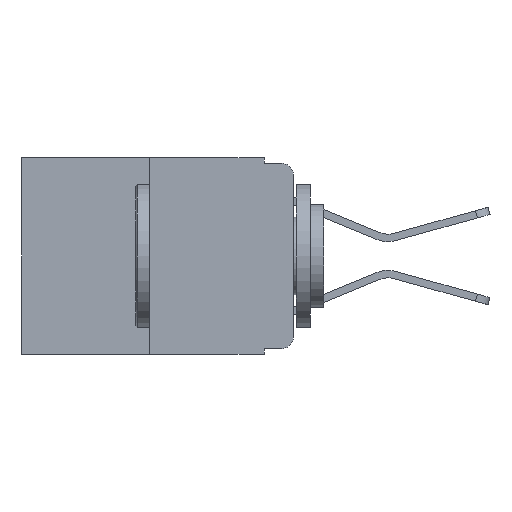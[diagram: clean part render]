
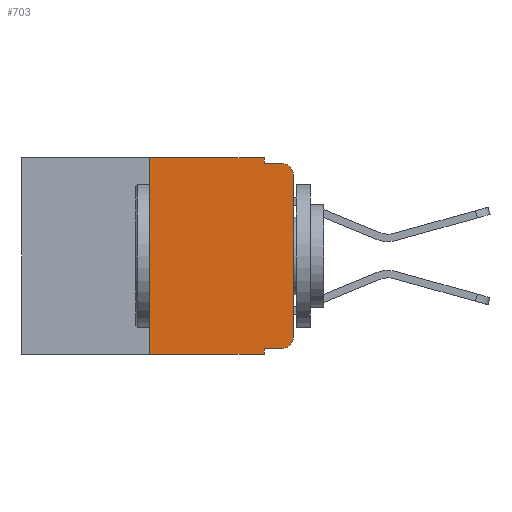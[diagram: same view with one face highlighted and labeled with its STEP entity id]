
A CAD part, left-side view. The second image highlights one B-rep face of the part: STEP entity #703.
In plain terms, the highlighted planar face has unit normal (-1, 0, 0).
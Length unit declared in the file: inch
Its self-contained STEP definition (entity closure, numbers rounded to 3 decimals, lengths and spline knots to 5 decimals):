
#100 = EDGE_CURVE ( 'NONE', #8835, #6657, #6032, .T. ) ;
#194 = DIRECTION ( 'NONE',  ( 0., 0., -1. ) ) ;
#227 = AXIS2_PLACEMENT_3D ( 'NONE', #9845, #1413, #9112 ) ;
#555 = LINE ( 'NONE', #8136, #9155 ) ;
#602 = LINE ( 'NONE', #9865, #4191 ) ;
#703 = ADVANCED_FACE ( 'NONE', ( #5547 ), #7226, .F. ) ;
#953 = VERTEX_POINT ( 'NONE', #3300 ) ;
#1245 = LINE ( 'NONE', #5343, #3093 ) ;
#1413 = DIRECTION ( 'NONE',  ( 1., 0., 0. ) ) ;
#1449 = VERTEX_POINT ( 'NONE', #7478 ) ;
#1774 = EDGE_CURVE ( 'NONE', #4949, #953, #2512, .T. ) ;
#1787 = CARTESIAN_POINT ( 'NONE',  ( 0., 0.051, 0. ) ) ;
#2020 = CARTESIAN_POINT ( 'NONE',  ( 0., 0., -0.313 ) ) ;
#2219 = AXIS2_PLACEMENT_3D ( 'NONE', #10643, #3145, #2368 ) ;
#2368 = DIRECTION ( 'NONE',  ( 0., 0., -1. ) ) ;
#2512 = LINE ( 'NONE', #8543, #6985 ) ;
#2522 = ORIENTED_EDGE ( 'NONE', *, *, #10010, .T. ) ;
#2546 = ORIENTED_EDGE ( 'NONE', *, *, #100, .F. ) ;
#2639 = CARTESIAN_POINT ( 'NONE',  ( 0., 0.02, -0.333 ) ) ;
#2897 = ORIENTED_EDGE ( 'NONE', *, *, #1774, .F. ) ;
#2967 = CARTESIAN_POINT ( 'NONE',  ( 0., 0.051, -0.01 ) ) ;
#3084 = LINE ( 'NONE', #6275, #6816 ) ;
#3093 = VECTOR ( 'NONE', #8728, 39.37008 ) ;
#3098 = DIRECTION ( 'NONE',  ( 0., -1., 0. ) ) ;
#3121 = VERTEX_POINT ( 'NONE', #2639 ) ;
#3131 = DIRECTION ( 'NONE',  ( 0., -1., 0. ) ) ;
#3145 = DIRECTION ( 'NONE',  ( -1., 0., 0. ) ) ;
#3300 = CARTESIAN_POINT ( 'NONE',  ( 0., 0.25, 0. ) ) ;
#3340 = EDGE_CURVE ( 'NONE', #6657, #1449, #10730, .T. ) ;
#3494 = LINE ( 'NONE', #5086, #8949 ) ;
#3714 = VERTEX_POINT ( 'NONE', #6875 ) ;
#3865 = DIRECTION ( 'NONE',  ( 0., -1., 0. ) ) ;
#4146 = CARTESIAN_POINT ( 'NONE',  ( 0., 0.051, -0.01 ) ) ;
#4191 = VECTOR ( 'NONE', #3098, 39.37008 ) ;
#4493 = ORIENTED_EDGE ( 'NONE', *, *, #6870, .F. ) ;
#4596 = VECTOR ( 'NONE', #194, 39.37008 ) ;
#4863 = VECTOR ( 'NONE', #3131, 39.37008 ) ;
#4949 = VERTEX_POINT ( 'NONE', #7816 ) ;
#5086 = CARTESIAN_POINT ( 'NONE',  ( 0., 0.051, 0. ) ) ;
#5343 = CARTESIAN_POINT ( 'NONE',  ( 0., 0.473, -0.343 ) ) ;
#5416 = AXIS2_PLACEMENT_3D ( 'NONE', #8142, #9871, #9083 ) ;
#5547 = FACE_OUTER_BOUND ( 'NONE', #9544, .T. ) ;
#5873 = DIRECTION ( 'NONE',  ( 0., 0., 1. ) ) ;
#5999 = CARTESIAN_POINT ( 'NONE',  ( 0., 0.051, -0.333 ) ) ;
#6032 = LINE ( 'NONE', #1787, #4596 ) ;
#6275 = CARTESIAN_POINT ( 'NONE',  ( 0., 0.051, -0.333 ) ) ;
#6484 = ORIENTED_EDGE ( 'NONE', *, *, #3340, .F. ) ;
#6657 = VERTEX_POINT ( 'NONE', #4146 ) ;
#6816 = VECTOR ( 'NONE', #3865, 39.37008 ) ;
#6857 = DIRECTION ( 'NONE',  ( 0., 0., -1. ) ) ;
#6870 = EDGE_CURVE ( 'NONE', #953, #8835, #602, .T. ) ;
#6875 = CARTESIAN_POINT ( 'NONE',  ( 0., 0., -0.03 ) ) ;
#6922 = EDGE_CURVE ( 'NONE', #8909, #3714, #555, .T. ) ;
#6963 = ORIENTED_EDGE ( 'NONE', *, *, #10040, .T. ) ;
#6985 = VECTOR ( 'NONE', #5873, 39.37008 ) ;
#7226 = PLANE ( 'NONE',  #227 ) ;
#7411 = CARTESIAN_POINT ( 'NONE',  ( 0., 0.051, -0.343 ) ) ;
#7478 = CARTESIAN_POINT ( 'NONE',  ( 0., 0.02, -0.01 ) ) ;
#7816 = CARTESIAN_POINT ( 'NONE',  ( 0., 0.25, -0.343 ) ) ;
#7962 = EDGE_CURVE ( 'NONE', #9827, #8265, #3494, .T. ) ;
#8136 = CARTESIAN_POINT ( 'NONE',  ( 0., 0., 0. ) ) ;
#8142 = CARTESIAN_POINT ( 'NONE',  ( 0., 0.02, -0.03 ) ) ;
#8265 = VERTEX_POINT ( 'NONE', #7411 ) ;
#8513 = CARTESIAN_POINT ( 'NONE',  ( 0., 0.051, 0. ) ) ;
#8543 = CARTESIAN_POINT ( 'NONE',  ( 0., 0.25, 0. ) ) ;
#8622 = EDGE_CURVE ( 'NONE', #9827, #3121, #3084, .T. ) ;
#8694 = ORIENTED_EDGE ( 'NONE', *, *, #6922, .T. ) ;
#8728 = DIRECTION ( 'NONE',  ( 0., -1., 0. ) ) ;
#8835 = VERTEX_POINT ( 'NONE', #8513 ) ;
#8909 = VERTEX_POINT ( 'NONE', #2020 ) ;
#8931 = CIRCLE ( 'NONE', #2219, 0.02 ) ;
#8949 = VECTOR ( 'NONE', #6857, 39.37008 ) ;
#9083 = DIRECTION ( 'NONE',  ( 0., 0., -1. ) ) ;
#9112 = DIRECTION ( 'NONE',  ( 0., 0., -1. ) ) ;
#9155 = VECTOR ( 'NONE', #10761, 39.37008 ) ;
#9311 = ORIENTED_EDGE ( 'NONE', *, *, #7962, .F. ) ;
#9439 = EDGE_CURVE ( 'NONE', #3714, #1449, #9681, .T. ) ;
#9544 = EDGE_LOOP ( 'NONE', ( #8694, #10514, #6484, #2546, #4493, #2897, #2522, #9311, #9593, #6963 ) ) ;
#9593 = ORIENTED_EDGE ( 'NONE', *, *, #8622, .T. ) ;
#9681 = CIRCLE ( 'NONE', #5416, 0.02 ) ;
#9827 = VERTEX_POINT ( 'NONE', #5999 ) ;
#9845 = CARTESIAN_POINT ( 'NONE',  ( 0., 0.473, 0. ) ) ;
#9865 = CARTESIAN_POINT ( 'NONE',  ( 0., 0.473, 0. ) ) ;
#9871 = DIRECTION ( 'NONE',  ( -1., 0., 0. ) ) ;
#10010 = EDGE_CURVE ( 'NONE', #4949, #8265, #1245, .T. ) ;
#10040 = EDGE_CURVE ( 'NONE', #3121, #8909, #8931, .T. ) ;
#10514 = ORIENTED_EDGE ( 'NONE', *, *, #9439, .T. ) ;
#10643 = CARTESIAN_POINT ( 'NONE',  ( 0., 0.02, -0.313 ) ) ;
#10730 = LINE ( 'NONE', #2967, #4863 ) ;
#10761 = DIRECTION ( 'NONE',  ( 0., 0., 1. ) ) ;
